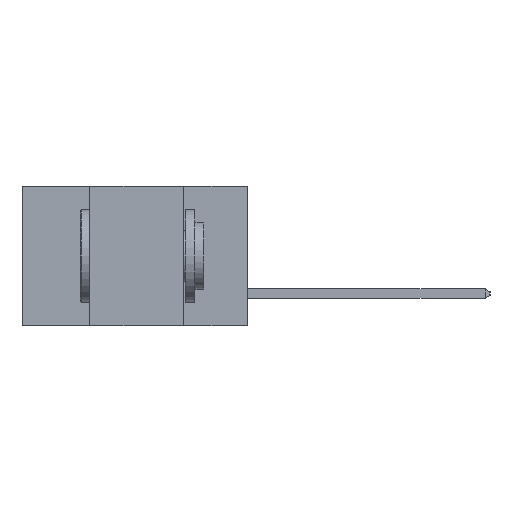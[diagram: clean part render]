
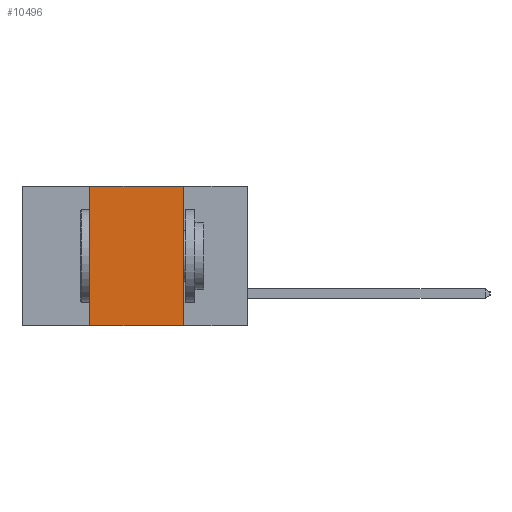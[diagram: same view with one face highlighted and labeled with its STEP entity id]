
A CAD part, left-side view. The second image highlights one B-rep face of the part: STEP entity #10496.
In plain terms, the highlighted planar face has unit normal (-1, 0, 0).
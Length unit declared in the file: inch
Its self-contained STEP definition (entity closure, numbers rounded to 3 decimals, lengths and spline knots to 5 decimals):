
#51 = VECTOR ( 'NONE', #6600, 39.37008 ) ;
#433 = CARTESIAN_POINT ( 'NONE',  ( 0., 0.17, 0. ) ) ;
#1562 = DIRECTION ( 'NONE',  ( 1., 0., 0. ) ) ;
#1950 = VERTEX_POINT ( 'NONE', #29313 ) ;
#2435 = CARTESIAN_POINT ( 'NONE',  ( 0., 0.42, 0. ) ) ;
#5437 = FACE_OUTER_BOUND ( 'NONE', #19327, .T. ) ;
#5665 = EDGE_CURVE ( 'NONE', #13266, #24923, #7917, .T. ) ;
#6600 = DIRECTION ( 'NONE',  ( 0., -1., 0. ) ) ;
#7917 = LINE ( 'NONE', #27820, #12762 ) ;
#8252 = CARTESIAN_POINT ( 'NONE',  ( 0., 0.42, 0. ) ) ;
#8390 = VERTEX_POINT ( 'NONE', #16793 ) ;
#8468 = LINE ( 'NONE', #433, #14063 ) ;
#9236 = EDGE_CURVE ( 'NONE', #24923, #1950, #8468, .T. ) ;
#10496 = ADVANCED_FACE ( 'NONE', ( #5437 ), #27676, .F. ) ;
#12762 = VECTOR ( 'NONE', #29695, 39.37008 ) ;
#13266 = VERTEX_POINT ( 'NONE', #8252 ) ;
#14063 = VECTOR ( 'NONE', #21889, 39.37008 ) ;
#14318 = ORIENTED_EDGE ( 'NONE', *, *, #9236, .F. ) ;
#15422 = ORIENTED_EDGE ( 'NONE', *, *, #28865, .T. ) ;
#16793 = CARTESIAN_POINT ( 'NONE',  ( 0., 0.42, -0.37 ) ) ;
#18295 = DIRECTION ( 'NONE',  ( 0., 0., -1. ) ) ;
#19327 = EDGE_LOOP ( 'NONE', ( #14318, #25231, #22046, #15422 ) ) ;
#19702 = CARTESIAN_POINT ( 'NONE',  ( 0., 0.17, 0. ) ) ;
#19850 = LINE ( 'NONE', #23194, #51 ) ;
#21889 = DIRECTION ( 'NONE',  ( 0., 0., -1. ) ) ;
#22046 = ORIENTED_EDGE ( 'NONE', *, *, #30438, .F. ) ;
#22340 = LINE ( 'NONE', #2435, #27899 ) ;
#23194 = CARTESIAN_POINT ( 'NONE',  ( 0., 0.6, -0.37 ) ) ;
#23863 = DIRECTION ( 'NONE',  ( 0., 0., 1. ) ) ;
#24923 = VERTEX_POINT ( 'NONE', #19702 ) ;
#25045 = AXIS2_PLACEMENT_3D ( 'NONE', #30057, #1562, #18295 ) ;
#25231 = ORIENTED_EDGE ( 'NONE', *, *, #5665, .F. ) ;
#27676 = PLANE ( 'NONE',  #25045 ) ;
#27820 = CARTESIAN_POINT ( 'NONE',  ( 0., 0.6, 0. ) ) ;
#27899 = VECTOR ( 'NONE', #23863, 39.37008 ) ;
#28865 = EDGE_CURVE ( 'NONE', #8390, #1950, #19850, .T. ) ;
#29313 = CARTESIAN_POINT ( 'NONE',  ( 0., 0.17, -0.37 ) ) ;
#29695 = DIRECTION ( 'NONE',  ( 0., -1., 0. ) ) ;
#30057 = CARTESIAN_POINT ( 'NONE',  ( 0., 0.6, 0. ) ) ;
#30438 = EDGE_CURVE ( 'NONE', #8390, #13266, #22340, .T. ) ;
